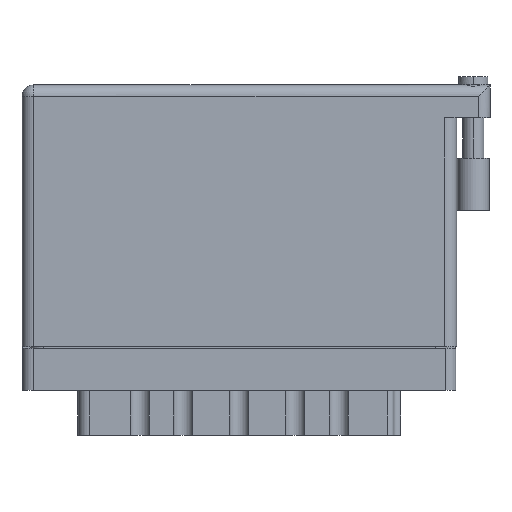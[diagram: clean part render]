
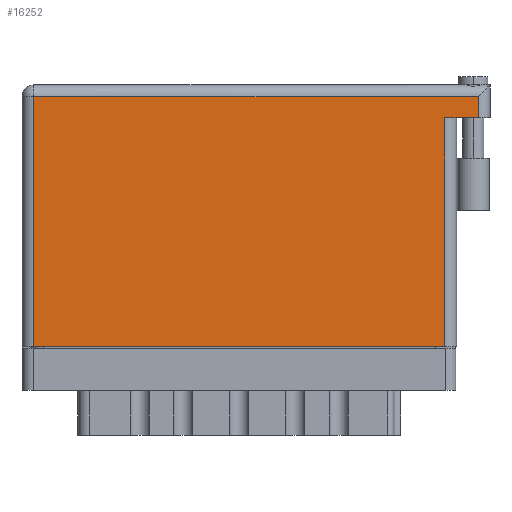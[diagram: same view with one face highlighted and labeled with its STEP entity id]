
A CAD part, front view. The second image highlights one B-rep face of the part: STEP entity #16252.
In plain terms, the highlighted face is planar.
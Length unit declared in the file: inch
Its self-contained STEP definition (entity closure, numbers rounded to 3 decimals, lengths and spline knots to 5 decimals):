
#513 = ORIENTED_EDGE ( 'NONE', *, *, #20617, .F. ) ;
#1036 = LINE ( 'NONE', #7959, #24234 ) ;
#1682 = VECTOR ( 'NONE', #30123, 39.37008 ) ;
#2633 = VECTOR ( 'NONE', #26235, 39.37008 ) ;
#3960 = CARTESIAN_POINT ( 'NONE',  ( 0., 1.496, 0. ) ) ;
#5185 = EDGE_CURVE ( 'NONE', #20883, #32858, #29023, .T. ) ;
#5811 = CARTESIAN_POINT ( 'NONE',  ( 0., 1.566, 0. ) ) ;
#6196 = CARTESIAN_POINT ( 'NONE',  ( 0.07, 1.496, 0. ) ) ;
#7036 = VERTEX_POINT ( 'NONE', #38437 ) ;
#7338 = EDGE_LOOP ( 'NONE', ( #16832, #23180, #513, #32871, #11415, #47503 ) ) ;
#7784 = CARTESIAN_POINT ( 'NONE',  ( 2.73, 1.496, 0. ) ) ;
#7959 = CARTESIAN_POINT ( 'NONE',  ( 2.8, 1.369, 0. ) ) ;
#9210 = CARTESIAN_POINT ( 'NONE',  ( 2.53, 1.369, 0. ) ) ;
#10178 = EDGE_CURVE ( 'NONE', #7036, #23432, #10316, .T. ) ;
#10316 = LINE ( 'NONE', #21898, #2633 ) ;
#11018 = LINE ( 'NONE', #3960, #47921 ) ;
#11252 = DIRECTION ( 'NONE',  ( -1., 0., 0. ) ) ;
#11415 = ORIENTED_EDGE ( 'NONE', *, *, #43004, .T. ) ;
#11444 = DIRECTION ( 'NONE',  ( 0., -1., 0. ) ) ;
#11767 = CARTESIAN_POINT ( 'NONE',  ( 0.07, 0., 0. ) ) ;
#12333 = VERTEX_POINT ( 'NONE', #6196 ) ;
#12470 = AXIS2_PLACEMENT_3D ( 'NONE', #5811, #28772, #39915 ) ;
#13407 = PLANE ( 'NONE',  #12470 ) ;
#15343 = FACE_OUTER_BOUND ( 'NONE', #7338, .T. ) ;
#16252 = ADVANCED_FACE ( 'NONE', ( #15343 ), #13407, .F. ) ;
#16832 = ORIENTED_EDGE ( 'NONE', *, *, #38347, .T. ) ;
#18624 = CARTESIAN_POINT ( 'NONE',  ( 2.73, 1.566, 0. ) ) ;
#20438 = LINE ( 'NONE', #11767, #27607 ) ;
#20617 = EDGE_CURVE ( 'NONE', #20883, #23432, #1036, .T. ) ;
#20883 = VERTEX_POINT ( 'NONE', #43529 ) ;
#21189 = LINE ( 'NONE', #34372, #33159 ) ;
#21898 = CARTESIAN_POINT ( 'NONE',  ( 2.53, 1.369, 0. ) ) ;
#23180 = ORIENTED_EDGE ( 'NONE', *, *, #10178, .T. ) ;
#23432 = VERTEX_POINT ( 'NONE', #9210 ) ;
#23546 = DIRECTION ( 'NONE',  ( 1., 0., 0. ) ) ;
#24234 = VECTOR ( 'NONE', #31079, 39.37008 ) ;
#26039 = VERTEX_POINT ( 'NONE', #28326 ) ;
#26235 = DIRECTION ( 'NONE',  ( 0., 1., 0. ) ) ;
#27607 = VECTOR ( 'NONE', #11444, 39.37008 ) ;
#28326 = CARTESIAN_POINT ( 'NONE',  ( 0.07, 0., 0. ) ) ;
#28772 = DIRECTION ( 'NONE',  ( 0., 0., -1. ) ) ;
#29023 = LINE ( 'NONE', #18624, #1682 ) ;
#30123 = DIRECTION ( 'NONE',  ( 0., 1., 0. ) ) ;
#31079 = DIRECTION ( 'NONE',  ( -1., 0., 0. ) ) ;
#32858 = VERTEX_POINT ( 'NONE', #7784 ) ;
#32871 = ORIENTED_EDGE ( 'NONE', *, *, #5185, .T. ) ;
#33159 = VECTOR ( 'NONE', #23546, 39.37008 ) ;
#34372 = CARTESIAN_POINT ( 'NONE',  ( 0., 0., 0. ) ) ;
#38347 = EDGE_CURVE ( 'NONE', #26039, #7036, #21189, .T. ) ;
#38437 = CARTESIAN_POINT ( 'NONE',  ( 2.53, 0., 0. ) ) ;
#39915 = DIRECTION ( 'NONE',  ( -1., 0., 0. ) ) ;
#43004 = EDGE_CURVE ( 'NONE', #32858, #12333, #11018, .T. ) ;
#43529 = CARTESIAN_POINT ( 'NONE',  ( 2.73, 1.369, 0. ) ) ;
#45656 = EDGE_CURVE ( 'NONE', #12333, #26039, #20438, .T. ) ;
#47503 = ORIENTED_EDGE ( 'NONE', *, *, #45656, .T. ) ;
#47921 = VECTOR ( 'NONE', #11252, 39.37008 ) ;
